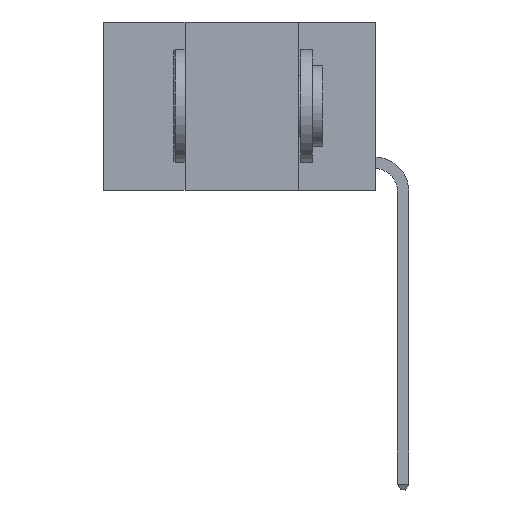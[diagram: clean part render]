
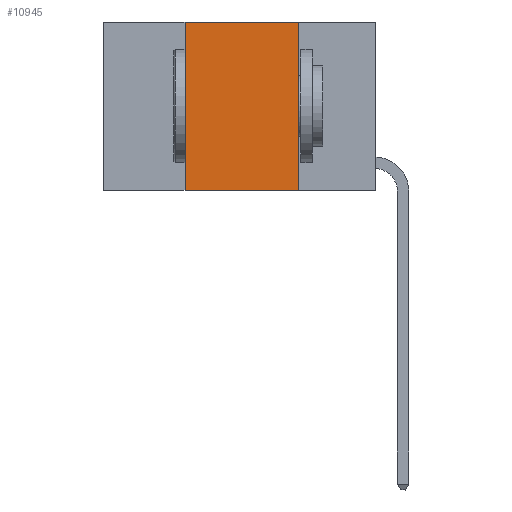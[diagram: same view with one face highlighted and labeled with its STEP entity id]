
A CAD part, left-side view. The second image highlights one B-rep face of the part: STEP entity #10945.
In plain terms, the highlighted planar face has unit normal (-1, 0, 0).
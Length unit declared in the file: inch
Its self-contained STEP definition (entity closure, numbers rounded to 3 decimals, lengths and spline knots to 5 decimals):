
#365 = VERTEX_POINT ( 'NONE', #11308 ) ;
#873 = FACE_OUTER_BOUND ( 'NONE', #11959, .T. ) ;
#1073 = DIRECTION ( 'NONE',  ( 0., 0., 1. ) ) ;
#1094 = DIRECTION ( 'NONE',  ( 0., 0., -1. ) ) ;
#1151 = LINE ( 'NONE', #5895, #5104 ) ;
#1768 = EDGE_CURVE ( 'NONE', #13098, #8868, #1151, .T. ) ;
#2285 = DIRECTION ( 'NONE',  ( 1., 0., 0. ) ) ;
#2493 = DIRECTION ( 'NONE',  ( 0., -1., 0. ) ) ;
#3128 = VECTOR ( 'NONE', #1073, 39.37008 ) ;
#3709 = CARTESIAN_POINT ( 'NONE',  ( 0., 0.17, -0.37 ) ) ;
#4568 = CARTESIAN_POINT ( 'NONE',  ( 0., 0.42, -0.37 ) ) ;
#5104 = VECTOR ( 'NONE', #2493, 39.37008 ) ;
#5132 = EDGE_CURVE ( 'NONE', #365, #8868, #10147, .T. ) ;
#5313 = VERTEX_POINT ( 'NONE', #8457 ) ;
#5648 = VECTOR ( 'NONE', #6817, 39.37008 ) ;
#5895 = CARTESIAN_POINT ( 'NONE',  ( 0., 0.6, -0.37 ) ) ;
#6817 = DIRECTION ( 'NONE',  ( 0., 0., -1. ) ) ;
#6950 = LINE ( 'NONE', #11849, #3128 ) ;
#7049 = VECTOR ( 'NONE', #8095, 39.37008 ) ;
#7158 = ORIENTED_EDGE ( 'NONE', *, *, #5132, .F. ) ;
#8095 = DIRECTION ( 'NONE',  ( 0., -1., 0. ) ) ;
#8284 = ORIENTED_EDGE ( 'NONE', *, *, #14494, .F. ) ;
#8457 = CARTESIAN_POINT ( 'NONE',  ( 0., 0.42, 0. ) ) ;
#8652 = ORIENTED_EDGE ( 'NONE', *, *, #14602, .F. ) ;
#8868 = VERTEX_POINT ( 'NONE', #3709 ) ;
#8922 = AXIS2_PLACEMENT_3D ( 'NONE', #12793, #2285, #1094 ) ;
#9597 = LINE ( 'NONE', #14313, #7049 ) ;
#10147 = LINE ( 'NONE', #12850, #5648 ) ;
#10945 = ADVANCED_FACE ( 'NONE', ( #873 ), #12570, .F. ) ;
#11308 = CARTESIAN_POINT ( 'NONE',  ( 0., 0.17, 0. ) ) ;
#11849 = CARTESIAN_POINT ( 'NONE',  ( 0., 0.42, 0. ) ) ;
#11959 = EDGE_LOOP ( 'NONE', ( #7158, #8652, #8284, #14747 ) ) ;
#12570 = PLANE ( 'NONE',  #8922 ) ;
#12793 = CARTESIAN_POINT ( 'NONE',  ( 0., 0.6, 0. ) ) ;
#12850 = CARTESIAN_POINT ( 'NONE',  ( 0., 0.17, 0. ) ) ;
#13098 = VERTEX_POINT ( 'NONE', #4568 ) ;
#14313 = CARTESIAN_POINT ( 'NONE',  ( 0., 0.6, 0. ) ) ;
#14494 = EDGE_CURVE ( 'NONE', #13098, #5313, #6950, .T. ) ;
#14602 = EDGE_CURVE ( 'NONE', #5313, #365, #9597, .T. ) ;
#14747 = ORIENTED_EDGE ( 'NONE', *, *, #1768, .T. ) ;
